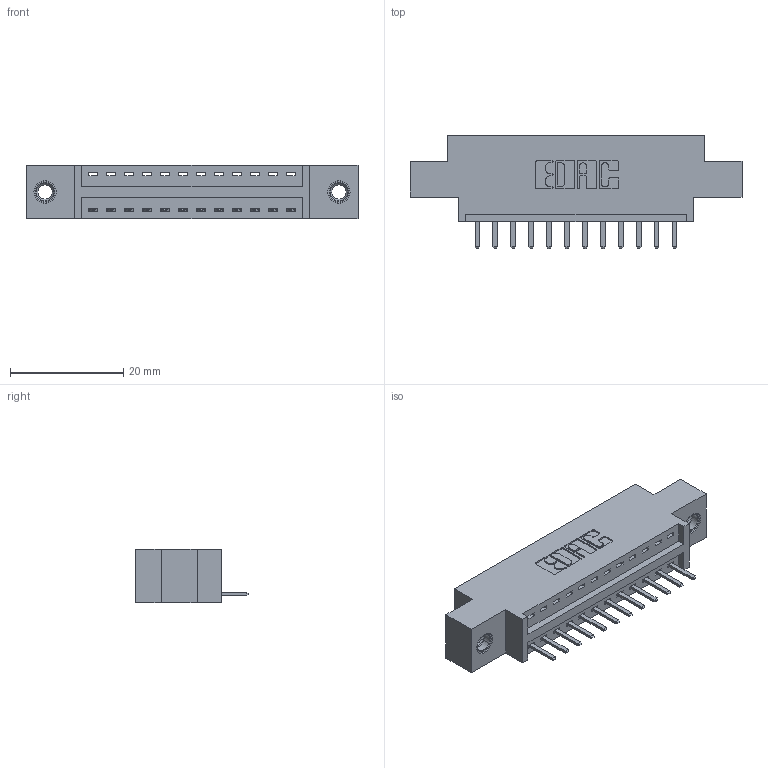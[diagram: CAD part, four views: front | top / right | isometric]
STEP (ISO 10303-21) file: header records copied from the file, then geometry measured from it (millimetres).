
FILE_DESCRIPTION (( 'STEP AP203' ), '1' );
FILE_NAME ('396-012-520-607.STEP', '2019-10-26T15:16:54', ( '' ), ( '' ), 'SwSTEP 2.0', 'SolidWorks 2016', '' );
FILE_SCHEMA (( 'CONFIG_CONTROL_DESIGN' ));
Length unit declared in the file: inch
Products named in the file (4): 345-292-001_345-293-120; 396-012-520-607; 345-250-001_345-250-005-103; 346 Part_0.170 Offset - 0.156 Dia-TI
Assembly tree (15 placements, depth 2):
  396-012-520-607
    346 Part_0.170 Offset - 0.156 Dia-TI
    345-292-001_345-293-120  x12
    345-250-001_345-250-005-103  x2
Bounding box: 58.67 x 20.02 x 9.4 mm (x, y, z)
Volume: 5207.1 mm3; surface area: 6264.2 mm2
Topology: 15 solids, 15 shells, 930 faces, 2685 edges, 1750 vertices
Faces by surface type: plane 616, cylinder 298, cone 12, torus 4
Entity records: 12918 total; most frequent: CARTESIAN_POINT 2219, ORIENTED_EDGE 2146, DIRECTION 2007, EDGE_CURVE 1073, LINE 869, VECTOR 869, VERTEX_POINT 708, AXIS2_PLACEMENT_3D 569
